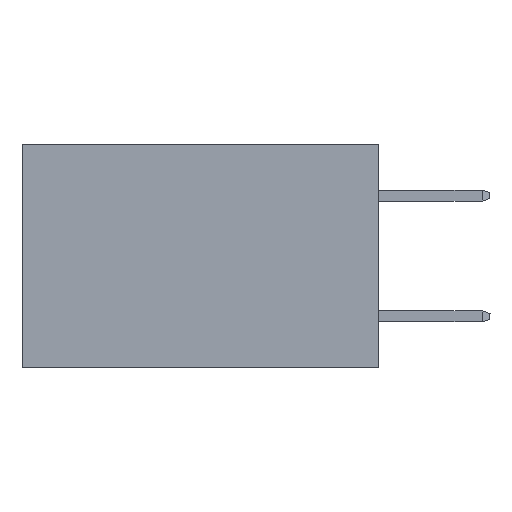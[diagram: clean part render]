
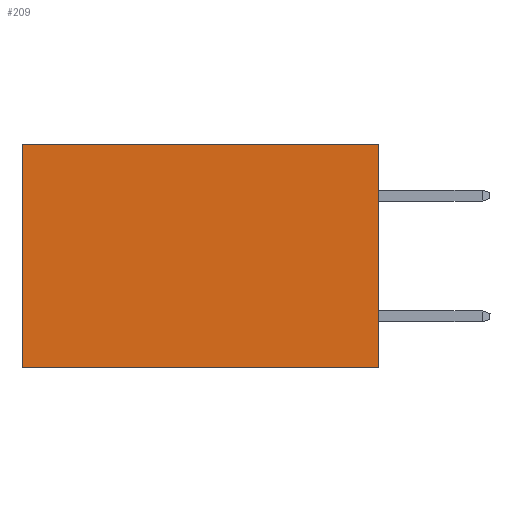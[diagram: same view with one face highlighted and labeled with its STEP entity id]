
A CAD part, left-side view. The second image highlights one B-rep face of the part: STEP entity #209.
In plain terms, the highlighted planar face has unit normal (-1, 0, 0).
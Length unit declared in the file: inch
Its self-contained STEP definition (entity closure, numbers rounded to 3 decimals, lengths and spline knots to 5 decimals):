
#209 = ADVANCED_FACE ( 'NONE', ( #14805 ), #10529, .F. ) ;
#361 = DIRECTION ( 'NONE',  ( 0., 0., -1. ) ) ;
#613 = CARTESIAN_POINT ( 'NONE',  ( 0.277, 0., -0.37 ) ) ;
#1937 = ORIENTED_EDGE ( 'NONE', *, *, #3305, .T. ) ;
#3244 = DIRECTION ( 'NONE',  ( 0., 1., 0. ) ) ;
#3305 = EDGE_CURVE ( 'NONE', #5024, #24806, #12152, .T. ) ;
#5024 = VERTEX_POINT ( 'NONE', #24035 ) ;
#6432 = CARTESIAN_POINT ( 'NONE',  ( 0.277, 0., -0.37 ) ) ;
#10183 = AXIS2_PLACEMENT_3D ( 'NONE', #6432, #11395, #19253 ) ;
#10529 = PLANE ( 'NONE',  #10183 ) ;
#11270 = EDGE_CURVE ( 'NONE', #5024, #16271, #11763, .T. ) ;
#11395 = DIRECTION ( 'NONE',  ( 1., 0., 0. ) ) ;
#11763 = LINE ( 'NONE', #613, #28834 ) ;
#12152 = LINE ( 'NONE', #20524, #24058 ) ;
#14805 = FACE_OUTER_BOUND ( 'NONE', #25433, .T. ) ;
#15415 = VERTEX_POINT ( 'NONE', #17528 ) ;
#16271 = VERTEX_POINT ( 'NONE', #18068 ) ;
#16471 = LINE ( 'NONE', #27170, #27587 ) ;
#16784 = CARTESIAN_POINT ( 'NONE',  ( 0.277, 0.59, 0. ) ) ;
#16973 = CARTESIAN_POINT ( 'NONE',  ( 0.277, 0., -0.37 ) ) ;
#17423 = EDGE_CURVE ( 'NONE', #24806, #15415, #16471, .T. ) ;
#17426 = ORIENTED_EDGE ( 'NONE', *, *, #24873, .F. ) ;
#17528 = CARTESIAN_POINT ( 'NONE',  ( 0.277, 0.59, -0.37 ) ) ;
#18068 = CARTESIAN_POINT ( 'NONE',  ( 0.277, 0., -0.37 ) ) ;
#18557 = ORIENTED_EDGE ( 'NONE', *, *, #11270, .F. ) ;
#19253 = DIRECTION ( 'NONE',  ( 0., 0., -1. ) ) ;
#19866 = ORIENTED_EDGE ( 'NONE', *, *, #17423, .T. ) ;
#20485 = VECTOR ( 'NONE', #3244, 39.37008 ) ;
#20524 = CARTESIAN_POINT ( 'NONE',  ( 0.277, 0., 0. ) ) ;
#21157 = DIRECTION ( 'NONE',  ( 0., 0., -1. ) ) ;
#21260 = DIRECTION ( 'NONE',  ( 0., 1., 0. ) ) ;
#24035 = CARTESIAN_POINT ( 'NONE',  ( 0.277, 0., 0. ) ) ;
#24058 = VECTOR ( 'NONE', #21260, 39.37008 ) ;
#24806 = VERTEX_POINT ( 'NONE', #16784 ) ;
#24873 = EDGE_CURVE ( 'NONE', #16271, #15415, #25707, .T. ) ;
#25433 = EDGE_LOOP ( 'NONE', ( #19866, #17426, #18557, #1937 ) ) ;
#25707 = LINE ( 'NONE', #16973, #20485 ) ;
#27170 = CARTESIAN_POINT ( 'NONE',  ( 0.277, 0.59, -0.37 ) ) ;
#27587 = VECTOR ( 'NONE', #361, 39.37008 ) ;
#28834 = VECTOR ( 'NONE', #21157, 39.37008 ) ;
